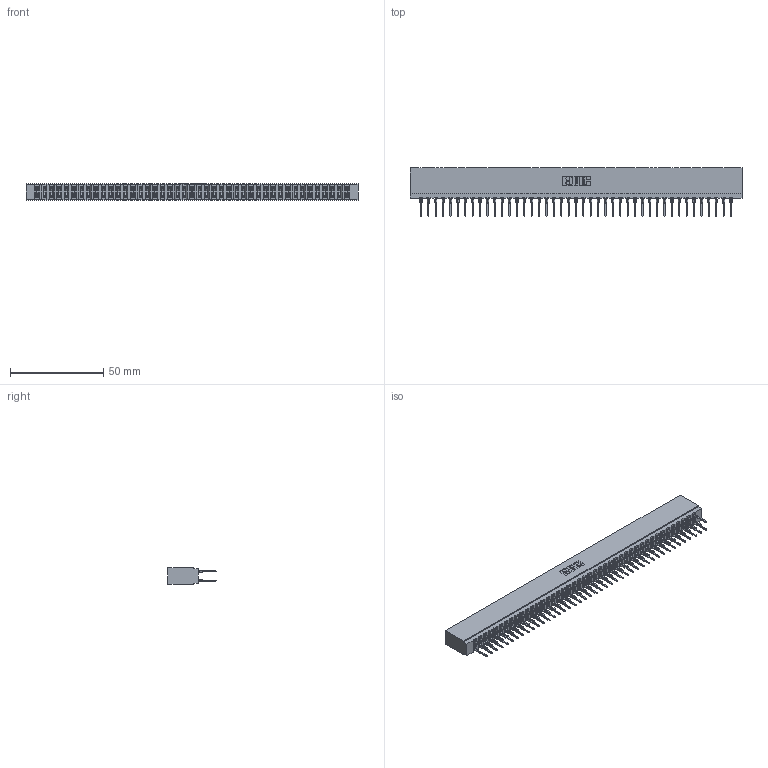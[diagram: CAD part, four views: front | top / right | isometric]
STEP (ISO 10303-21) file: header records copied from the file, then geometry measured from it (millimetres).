
FILE_DESCRIPTION (( 'STEP AP203' ), '1' );
FILE_NAME ('737-086-522-201.STEP', '2026-03-06T02:29:05', ( '' ), ( '' ), 'SwSTEP 2.0', 'SolidWorks 2023', '' );
FILE_SCHEMA (( 'CONFIG_CONTROL_DESIGN' ));
Length unit declared in the file: millimetre
Products named in the file (3): 737 Part_Insulator Option - 01; 745-292-001_522; 737-086-522-201
Assembly tree (87 placements, depth 2):
  737-086-522-201
    737 Part_Insulator Option - 01
    745-292-001_522  x86
Bounding box: 178.26 x 25.92 x 8.89 mm (x, y, z)
Volume: 17641.9 mm3; surface area: 26364.9 mm2
Topology: 87 solids, 87 shells, 7834 faces, 21067 edges, 13242 vertices
Faces by surface type: plane 4053, bspline 1720, cylinder 1545, torus 516
Entity records: 73641 total; most frequent: CARTESIAN_POINT 13287, ORIENTED_EDGE 12724, DIRECTION 11104, EDGE_CURVE 6362, LINE 5922, VECTOR 5922, VERTEX_POINT 4062, AXIS2_PLACEMENT_3D 2591
